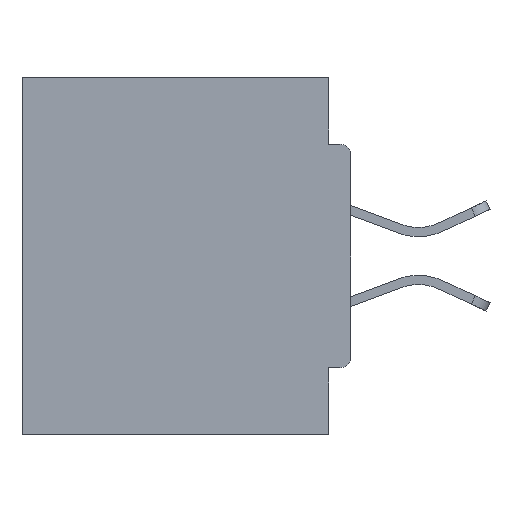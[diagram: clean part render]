
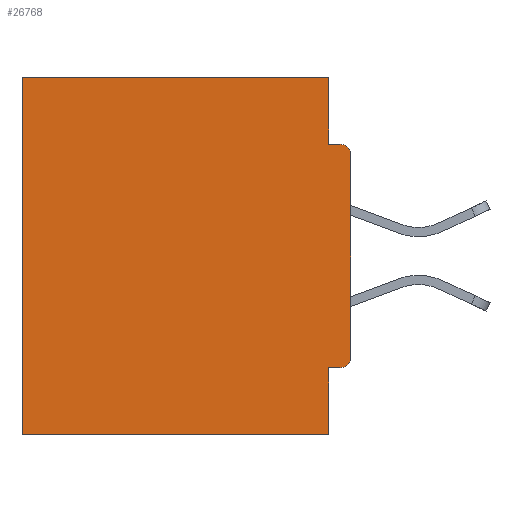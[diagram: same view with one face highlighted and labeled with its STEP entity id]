
A CAD part, left-side view. The second image highlights one B-rep face of the part: STEP entity #26768.
In plain terms, the highlighted planar face has unit normal (-1, 0, 0).
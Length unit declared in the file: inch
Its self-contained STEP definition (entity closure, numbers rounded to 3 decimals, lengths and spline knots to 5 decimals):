
#4 = DIRECTION ( 'NONE',  ( 0., 0., -1. ) ) ;
#604 = VECTOR ( 'NONE', #5725, 39.37008 ) ;
#620 = CARTESIAN_POINT ( 'NONE',  ( 0.298, 0.031, -0.5 ) ) ;
#924 = CARTESIAN_POINT ( 'NONE',  ( 0.298, 0., -0.5 ) ) ;
#1247 = VERTEX_POINT ( 'NONE', #10136 ) ;
#1615 = VERTEX_POINT ( 'NONE', #27108 ) ;
#1771 = VERTEX_POINT ( 'NONE', #21012 ) ;
#2495 = LINE ( 'NONE', #19517, #24550 ) ;
#2582 = EDGE_CURVE ( 'NONE', #1247, #8607, #22634, .T. ) ;
#2629 = EDGE_CURVE ( 'NONE', #21100, #10293, #30746, .T. ) ;
#3216 = CARTESIAN_POINT ( 'NONE',  ( 0.298, 0.031, -0.5 ) ) ;
#3337 = LINE ( 'NONE', #30801, #30030 ) ;
#3679 = CARTESIAN_POINT ( 'NONE',  ( 0.298, 0.015, -0.3915 ) ) ;
#4525 = CARTESIAN_POINT ( 'NONE',  ( 0.298, 0., 0. ) ) ;
#5534 = LINE ( 'NONE', #18201, #21783 ) ;
#5725 = DIRECTION ( 'NONE',  ( 0., 0., -1. ) ) ;
#6505 = ORIENTED_EDGE ( 'NONE', *, *, #19730, .F. ) ;
#7639 = AXIS2_PLACEMENT_3D ( 'NONE', #4525, #9289, #9510 ) ;
#7801 = CARTESIAN_POINT ( 'NONE',  ( 0.298, 0.015, -0.4065 ) ) ;
#7849 = ORIENTED_EDGE ( 'NONE', *, *, #24224, .F. ) ;
#8203 = CARTESIAN_POINT ( 'NONE',  ( 0.298, 0.031, 0. ) ) ;
#8307 = LINE ( 'NONE', #14963, #20639 ) ;
#8607 = VERTEX_POINT ( 'NONE', #20006 ) ;
#9182 = DIRECTION ( 'NONE',  ( -1., 0., 0. ) ) ;
#9289 = DIRECTION ( 'NONE',  ( 1., 0., 0. ) ) ;
#9290 = DIRECTION ( 'NONE',  ( 0., 0., -1. ) ) ;
#9510 = DIRECTION ( 'NONE',  ( 0., 0., -1. ) ) ;
#10012 = DIRECTION ( 'NONE',  ( 0., 1., 0. ) ) ;
#10136 = CARTESIAN_POINT ( 'NONE',  ( 0.298, 0., -0.1085 ) ) ;
#10176 = VERTEX_POINT ( 'NONE', #30614 ) ;
#10293 = VERTEX_POINT ( 'NONE', #14182 ) ;
#10603 = CARTESIAN_POINT ( 'NONE',  ( 0.298, 0.46, 0. ) ) ;
#10847 = DIRECTION ( 'NONE',  ( 0., 1., 0. ) ) ;
#10901 = VERTEX_POINT ( 'NONE', #7801 ) ;
#11378 = DIRECTION ( 'NONE',  ( 0., 0., -1. ) ) ;
#12672 = VERTEX_POINT ( 'NONE', #8203 ) ;
#12703 = EDGE_LOOP ( 'NONE', ( #20568, #26659, #7849, #27586, #26331, #30497, #6505, #14555, #27053, #26852 ) ) ;
#12906 = DIRECTION ( 'NONE',  ( 0., -1., 0. ) ) ;
#14182 = CARTESIAN_POINT ( 'NONE',  ( 0.298, 0.46, -0.5 ) ) ;
#14340 = CARTESIAN_POINT ( 'NONE',  ( 0.298, 0.46, 0. ) ) ;
#14555 = ORIENTED_EDGE ( 'NONE', *, *, #20207, .F. ) ;
#14963 = CARTESIAN_POINT ( 'NONE',  ( 0.298, 0., 0. ) ) ;
#17997 = CARTESIAN_POINT ( 'NONE',  ( 0.298, 0., -0.0935 ) ) ;
#18201 = CARTESIAN_POINT ( 'NONE',  ( 0.298, 0.031, -0.5 ) ) ;
#18202 = CARTESIAN_POINT ( 'NONE',  ( 0.298, 0.015, -0.1085 ) ) ;
#18845 = DIRECTION ( 'NONE',  ( 0., 0., -1. ) ) ;
#19005 = AXIS2_PLACEMENT_3D ( 'NONE', #3679, #23677, #11378 ) ;
#19288 = PLANE ( 'NONE',  #7639 ) ;
#19517 = CARTESIAN_POINT ( 'NONE',  ( 0.298, 0., -0.4065 ) ) ;
#19553 = VECTOR ( 'NONE', #10012, 39.37008 ) ;
#19730 = EDGE_CURVE ( 'NONE', #1771, #21100, #31889, .T. ) ;
#20006 = CARTESIAN_POINT ( 'NONE',  ( 0.298, 0.015, -0.0935 ) ) ;
#20207 = EDGE_CURVE ( 'NONE', #10901, #1771, #2495, .T. ) ;
#20568 = ORIENTED_EDGE ( 'NONE', *, *, #2582, .T. ) ;
#20639 = VECTOR ( 'NONE', #4, 39.37008 ) ;
#21012 = CARTESIAN_POINT ( 'NONE',  ( 0.298, 0.031, -0.4065 ) ) ;
#21100 = VERTEX_POINT ( 'NONE', #620 ) ;
#21783 = VECTOR ( 'NONE', #18845, 39.37008 ) ;
#22634 = CIRCLE ( 'NONE', #30344, 0.015 ) ;
#23314 = VERTEX_POINT ( 'NONE', #14340 ) ;
#23677 = DIRECTION ( 'NONE',  ( -1., 0., 0. ) ) ;
#24180 = LINE ( 'NONE', #17997, #26864 ) ;
#24224 = EDGE_CURVE ( 'NONE', #12672, #10176, #5534, .T. ) ;
#24550 = VECTOR ( 'NONE', #29573, 39.37008 ) ;
#24646 = VECTOR ( 'NONE', #30266, 39.37008 ) ;
#24996 = CIRCLE ( 'NONE', #19005, 0.015 ) ;
#25826 = FACE_OUTER_BOUND ( 'NONE', #12703, .T. ) ;
#26331 = ORIENTED_EDGE ( 'NONE', *, *, #27223, .T. ) ;
#26659 = ORIENTED_EDGE ( 'NONE', *, *, #29312, .F. ) ;
#26768 = ADVANCED_FACE ( 'NONE', ( #25826 ), #19288, .F. ) ;
#26852 = ORIENTED_EDGE ( 'NONE', *, *, #30061, .F. ) ;
#26864 = VECTOR ( 'NONE', #12906, 39.37008 ) ;
#27053 = ORIENTED_EDGE ( 'NONE', *, *, #28375, .T. ) ;
#27108 = CARTESIAN_POINT ( 'NONE',  ( 0.298, 0., -0.3915 ) ) ;
#27223 = EDGE_CURVE ( 'NONE', #23314, #10293, #30813, .T. ) ;
#27586 = ORIENTED_EDGE ( 'NONE', *, *, #28827, .T. ) ;
#28375 = EDGE_CURVE ( 'NONE', #10901, #1615, #24996, .T. ) ;
#28827 = EDGE_CURVE ( 'NONE', #12672, #23314, #3337, .T. ) ;
#29312 = EDGE_CURVE ( 'NONE', #10176, #8607, #24180, .T. ) ;
#29573 = DIRECTION ( 'NONE',  ( 0., 1., 0. ) ) ;
#30030 = VECTOR ( 'NONE', #10847, 39.37008 ) ;
#30061 = EDGE_CURVE ( 'NONE', #1247, #1615, #8307, .T. ) ;
#30266 = DIRECTION ( 'NONE',  ( 0., 0., -1. ) ) ;
#30344 = AXIS2_PLACEMENT_3D ( 'NONE', #18202, #9182, #9290 ) ;
#30497 = ORIENTED_EDGE ( 'NONE', *, *, #2629, .F. ) ;
#30614 = CARTESIAN_POINT ( 'NONE',  ( 0.298, 0.031, -0.0935 ) ) ;
#30746 = LINE ( 'NONE', #924, #19553 ) ;
#30801 = CARTESIAN_POINT ( 'NONE',  ( 0.298, 0., 0. ) ) ;
#30813 = LINE ( 'NONE', #10603, #24646 ) ;
#31889 = LINE ( 'NONE', #3216, #604 ) ;
